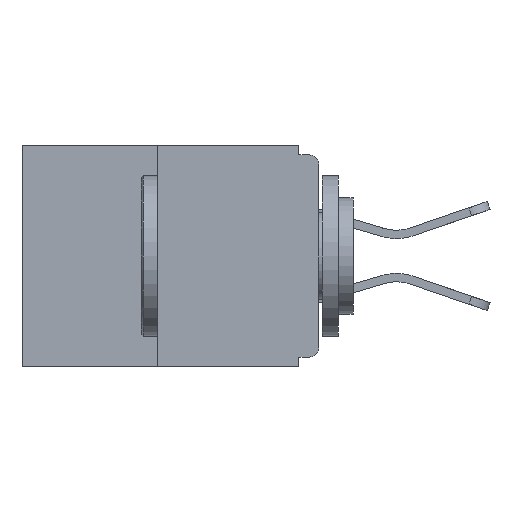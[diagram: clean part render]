
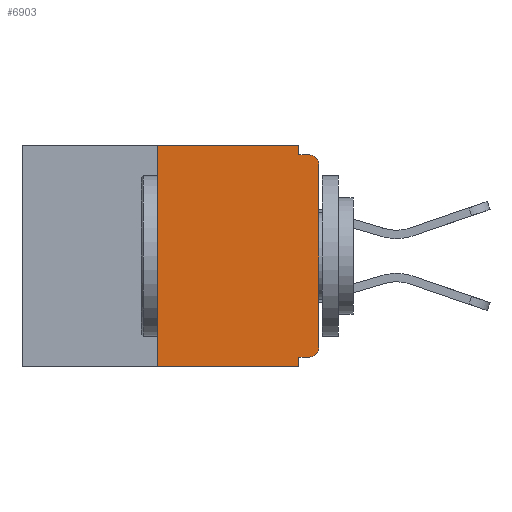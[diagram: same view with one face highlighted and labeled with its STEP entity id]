
A CAD part, left-side view. The second image highlights one B-rep face of the part: STEP entity #6903.
In plain terms, the highlighted planar face has unit normal (-1, 0, 0).
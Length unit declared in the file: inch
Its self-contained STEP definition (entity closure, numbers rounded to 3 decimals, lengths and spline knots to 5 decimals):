
#23 = EDGE_CURVE ( 'NONE', #7382, #3145, #317, .T. ) ;
#283 = EDGE_CURVE ( 'NONE', #4712, #10428, #14662, .T. ) ;
#317 = LINE ( 'NONE', #13370, #9479 ) ;
#841 = CARTESIAN_POINT ( 'NONE',  ( 0., 0.031, -0.343 ) ) ;
#868 = CARTESIAN_POINT ( 'NONE',  ( 0., 0.25, -0.343 ) ) ;
#1099 = CARTESIAN_POINT ( 'NONE',  ( 0., 0., -0.328 ) ) ;
#1144 = VECTOR ( 'NONE', #12504, 39.37008 ) ;
#1491 = EDGE_CURVE ( 'NONE', #14247, #7382, #13145, .T. ) ;
#1618 = FACE_OUTER_BOUND ( 'NONE', #12068, .T. ) ;
#1678 = CARTESIAN_POINT ( 'NONE',  ( 0., 0.015, -0.03 ) ) ;
#1783 = DIRECTION ( 'NONE',  ( 0., 0., -1. ) ) ;
#1808 = CARTESIAN_POINT ( 'NONE',  ( 0., 0.46, 0. ) ) ;
#1923 = VECTOR ( 'NONE', #8398, 39.37008 ) ;
#2880 = DIRECTION ( 'NONE',  ( 0., 0., -1. ) ) ;
#2959 = EDGE_CURVE ( 'NONE', #6286, #12671, #9379, .T. ) ;
#3022 = DIRECTION ( 'NONE',  ( 0., 0., 1. ) ) ;
#3145 = VERTEX_POINT ( 'NONE', #841 ) ;
#3191 = AXIS2_PLACEMENT_3D ( 'NONE', #8433, #7181, #10853 ) ;
#3298 = CARTESIAN_POINT ( 'NONE',  ( 0., 0., -0.03 ) ) ;
#3404 = LINE ( 'NONE', #13798, #1144 ) ;
#3510 = ORIENTED_EDGE ( 'NONE', *, *, #23, .F. ) ;
#3847 = ORIENTED_EDGE ( 'NONE', *, *, #12051, .F. ) ;
#3966 = CARTESIAN_POINT ( 'NONE',  ( 0., 0.25, 0. ) ) ;
#4392 = CIRCLE ( 'NONE', #4584, 0.015 ) ;
#4486 = EDGE_CURVE ( 'NONE', #14247, #4712, #6189, .T. ) ;
#4525 = ORIENTED_EDGE ( 'NONE', *, *, #4486, .T. ) ;
#4584 = AXIS2_PLACEMENT_3D ( 'NONE', #1678, #10053, #2880 ) ;
#4640 = CARTESIAN_POINT ( 'NONE',  ( 0., 0., -0.313 ) ) ;
#4712 = VERTEX_POINT ( 'NONE', #4640 ) ;
#5236 = ORIENTED_EDGE ( 'NONE', *, *, #1491, .F. ) ;
#5334 = ORIENTED_EDGE ( 'NONE', *, *, #283, .T. ) ;
#6017 = LINE ( 'NONE', #1808, #11255 ) ;
#6168 = CARTESIAN_POINT ( 'NONE',  ( 0., 0.015, -0.328 ) ) ;
#6189 = CIRCLE ( 'NONE', #9368, 0.015 ) ;
#6286 = VERTEX_POINT ( 'NONE', #868 ) ;
#6850 = VECTOR ( 'NONE', #9736, 39.37008 ) ;
#6903 = ADVANCED_FACE ( 'NONE', ( #1618 ), #9548, .F. ) ;
#7141 = CARTESIAN_POINT ( 'NONE',  ( 0., 0.031, -0.015 ) ) ;
#7181 = DIRECTION ( 'NONE',  ( 1., 0., 0. ) ) ;
#7382 = VERTEX_POINT ( 'NONE', #9875 ) ;
#7436 = EDGE_CURVE ( 'NONE', #6286, #3145, #13754, .T. ) ;
#7520 = DIRECTION ( 'NONE',  ( 0., 0., 1. ) ) ;
#7768 = CARTESIAN_POINT ( 'NONE',  ( 0., 0., 0. ) ) ;
#7865 = VECTOR ( 'NONE', #7520, 39.37008 ) ;
#7900 = DIRECTION ( 'NONE',  ( -1., 0., 0. ) ) ;
#8398 = DIRECTION ( 'NONE',  ( 0., 1., 0. ) ) ;
#8433 = CARTESIAN_POINT ( 'NONE',  ( 0., 0.46, 0. ) ) ;
#8486 = EDGE_CURVE ( 'NONE', #10428, #14840, #4392, .T. ) ;
#8523 = VECTOR ( 'NONE', #14156, 39.37008 ) ;
#8847 = DIRECTION ( 'NONE',  ( 0., -1., 0. ) ) ;
#8928 = ORIENTED_EDGE ( 'NONE', *, *, #2959, .F. ) ;
#9059 = ORIENTED_EDGE ( 'NONE', *, *, #10297, .F. ) ;
#9368 = AXIS2_PLACEMENT_3D ( 'NONE', #12537, #7900, #1783 ) ;
#9379 = LINE ( 'NONE', #3966, #7865 ) ;
#9453 = CARTESIAN_POINT ( 'NONE',  ( 0., 0.46, -0.343 ) ) ;
#9479 = VECTOR ( 'NONE', #12024, 39.37008 ) ;
#9545 = EDGE_CURVE ( 'NONE', #15107, #14840, #3404, .T. ) ;
#9548 = PLANE ( 'NONE',  #3191 ) ;
#9736 = DIRECTION ( 'NONE',  ( 0., 0., -1. ) ) ;
#9875 = CARTESIAN_POINT ( 'NONE',  ( 0., 0.031, -0.328 ) ) ;
#9885 = VERTEX_POINT ( 'NONE', #13771 ) ;
#10053 = DIRECTION ( 'NONE',  ( -1., 0., 0. ) ) ;
#10297 = EDGE_CURVE ( 'NONE', #12671, #9885, #6017, .T. ) ;
#10403 = VECTOR ( 'NONE', #3022, 39.37008 ) ;
#10428 = VERTEX_POINT ( 'NONE', #3298 ) ;
#10629 = LINE ( 'NONE', #14274, #6850 ) ;
#10853 = DIRECTION ( 'NONE',  ( 0., 0., -1. ) ) ;
#11255 = VECTOR ( 'NONE', #8847, 39.37008 ) ;
#12024 = DIRECTION ( 'NONE',  ( 0., 0., -1. ) ) ;
#12051 = EDGE_CURVE ( 'NONE', #9885, #15107, #10629, .T. ) ;
#12068 = EDGE_LOOP ( 'NONE', ( #9059, #8928, #13037, #3510, #5236, #4525, #5334, #13045, #13734, #3847 ) ) ;
#12289 = CARTESIAN_POINT ( 'NONE',  ( 0., 0.25, 0. ) ) ;
#12504 = DIRECTION ( 'NONE',  ( 0., -1., 0. ) ) ;
#12537 = CARTESIAN_POINT ( 'NONE',  ( 0., 0.015, -0.313 ) ) ;
#12671 = VERTEX_POINT ( 'NONE', #12289 ) ;
#13037 = ORIENTED_EDGE ( 'NONE', *, *, #7436, .T. ) ;
#13045 = ORIENTED_EDGE ( 'NONE', *, *, #8486, .T. ) ;
#13145 = LINE ( 'NONE', #1099, #1923 ) ;
#13370 = CARTESIAN_POINT ( 'NONE',  ( 0., 0.031, -0.343 ) ) ;
#13675 = CARTESIAN_POINT ( 'NONE',  ( 0., 0.015, -0.015 ) ) ;
#13734 = ORIENTED_EDGE ( 'NONE', *, *, #9545, .F. ) ;
#13754 = LINE ( 'NONE', #9453, #8523 ) ;
#13771 = CARTESIAN_POINT ( 'NONE',  ( 0., 0.031, 0. ) ) ;
#13798 = CARTESIAN_POINT ( 'NONE',  ( 0., 0., -0.015 ) ) ;
#14156 = DIRECTION ( 'NONE',  ( 0., -1., 0. ) ) ;
#14247 = VERTEX_POINT ( 'NONE', #6168 ) ;
#14274 = CARTESIAN_POINT ( 'NONE',  ( 0., 0.031, 0. ) ) ;
#14662 = LINE ( 'NONE', #7768, #10403 ) ;
#14840 = VERTEX_POINT ( 'NONE', #13675 ) ;
#15107 = VERTEX_POINT ( 'NONE', #7141 ) ;
